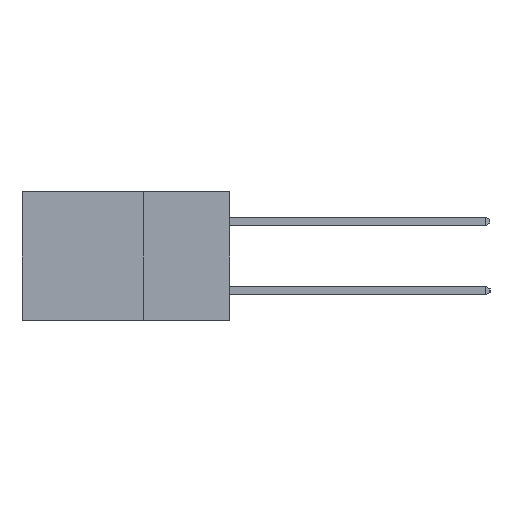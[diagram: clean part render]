
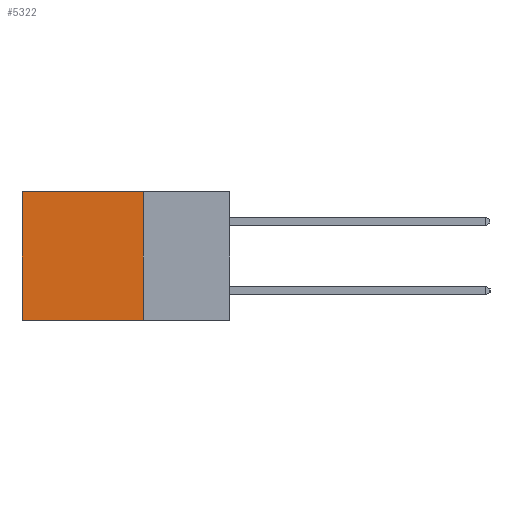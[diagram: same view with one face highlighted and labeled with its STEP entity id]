
A CAD part, left-side view. The second image highlights one B-rep face of the part: STEP entity #5322.
In plain terms, the highlighted planar face has unit normal (-1, 0, 0).
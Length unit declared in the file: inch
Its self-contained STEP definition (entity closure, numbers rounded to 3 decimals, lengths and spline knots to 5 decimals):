
#109 = ORIENTED_EDGE ( 'NONE', *, *, #14267, .T. ) ;
#521 = VERTEX_POINT ( 'NONE', #15472 ) ;
#811 = DIRECTION ( 'NONE',  ( 0., 0., -1. ) ) ;
#1469 = ORIENTED_EDGE ( 'NONE', *, *, #11848, .F. ) ;
#1704 = DIRECTION ( 'NONE',  ( 0., 1., 0. ) ) ;
#1762 = CARTESIAN_POINT ( 'NONE',  ( 0.2615, 0.25, -0.37 ) ) ;
#2469 = CARTESIAN_POINT ( 'NONE',  ( 0.2615, 0.25, 0. ) ) ;
#2595 = EDGE_LOOP ( 'NONE', ( #109, #1469, #14723, #6088 ) ) ;
#4251 = VECTOR ( 'NONE', #811, 39.37008 ) ;
#4662 = LINE ( 'NONE', #15115, #11044 ) ;
#4901 = FACE_OUTER_BOUND ( 'NONE', #2595, .T. ) ;
#5225 = DIRECTION ( 'NONE',  ( 0., 0., -1. ) ) ;
#5322 = ADVANCED_FACE ( 'NONE', ( #4901 ), #8885, .F. ) ;
#5393 = DIRECTION ( 'NONE',  ( 1., 0., 0. ) ) ;
#6088 = ORIENTED_EDGE ( 'NONE', *, *, #14636, .T. ) ;
#6267 = CARTESIAN_POINT ( 'NONE',  ( 0.2615, 0.25, -0.37 ) ) ;
#6338 = VERTEX_POINT ( 'NONE', #13605 ) ;
#6533 = VECTOR ( 'NONE', #1704, 39.37008 ) ;
#6676 = DIRECTION ( 'NONE',  ( 0., 0., -1. ) ) ;
#7639 = LINE ( 'NONE', #14879, #4251 ) ;
#7755 = EDGE_CURVE ( 'NONE', #9540, #8271, #7639, .T. ) ;
#8140 = CARTESIAN_POINT ( 'NONE',  ( 0.2615, 0.25, 0. ) ) ;
#8271 = VERTEX_POINT ( 'NONE', #12293 ) ;
#8564 = AXIS2_PLACEMENT_3D ( 'NONE', #6267, #5393, #5225 ) ;
#8790 = DIRECTION ( 'NONE',  ( 0., 1., 0. ) ) ;
#8885 = PLANE ( 'NONE',  #8564 ) ;
#9540 = VERTEX_POINT ( 'NONE', #8140 ) ;
#9634 = VECTOR ( 'NONE', #8790, 39.37008 ) ;
#10037 = LINE ( 'NONE', #2469, #9634 ) ;
#11044 = VECTOR ( 'NONE', #6676, 39.37008 ) ;
#11848 = EDGE_CURVE ( 'NONE', #8271, #6338, #13558, .T. ) ;
#12293 = CARTESIAN_POINT ( 'NONE',  ( 0.2615, 0.25, -0.37 ) ) ;
#13558 = LINE ( 'NONE', #1762, #6533 ) ;
#13605 = CARTESIAN_POINT ( 'NONE',  ( 0.2615, 0.6, -0.37 ) ) ;
#14267 = EDGE_CURVE ( 'NONE', #521, #6338, #4662, .T. ) ;
#14636 = EDGE_CURVE ( 'NONE', #9540, #521, #10037, .T. ) ;
#14723 = ORIENTED_EDGE ( 'NONE', *, *, #7755, .F. ) ;
#14879 = CARTESIAN_POINT ( 'NONE',  ( 0.2615, 0.25, -0.37 ) ) ;
#15115 = CARTESIAN_POINT ( 'NONE',  ( 0.2615, 0.6, -0.37 ) ) ;
#15472 = CARTESIAN_POINT ( 'NONE',  ( 0.2615, 0.6, 0. ) ) ;
